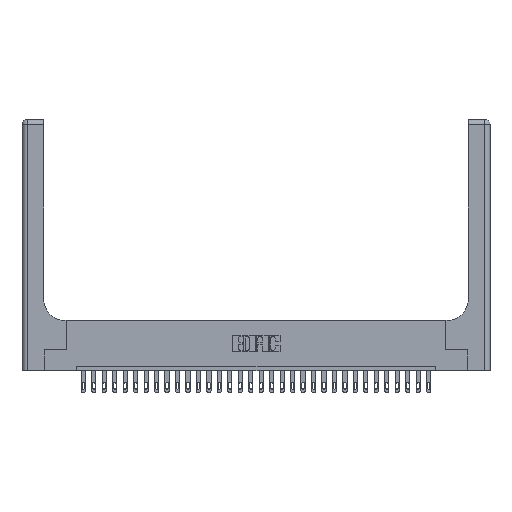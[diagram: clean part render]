
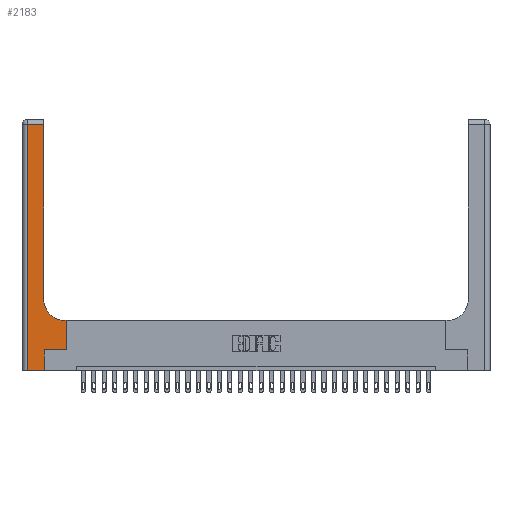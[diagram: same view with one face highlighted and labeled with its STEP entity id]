
A CAD part, top view. The second image highlights one B-rep face of the part: STEP entity #2183.
In plain terms, the highlighted planar face has unit normal (0, 0, 1).
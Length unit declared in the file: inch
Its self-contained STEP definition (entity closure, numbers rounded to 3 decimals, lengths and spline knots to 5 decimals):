
#355 = VERTEX_POINT ( 'NONE', #3595 ) ;
#551 = LINE ( 'NONE', #9182, #11327 ) ;
#972 = ORIENTED_EDGE ( 'NONE', *, *, #5209, .T. ) ;
#1092 = LINE ( 'NONE', #9715, #8685 ) ;
#1615 = VECTOR ( 'NONE', #13445, 39.37008 ) ;
#1952 = CARTESIAN_POINT ( 'NONE',  ( 0.528, 0.25, 0.37 ) ) ;
#2121 = VERTEX_POINT ( 'NONE', #25335 ) ;
#2130 = DIRECTION ( 'NONE',  ( 1., 0., 0. ) ) ;
#2183 = ADVANCED_FACE ( 'NONE', ( #14307 ), #10513, .F. ) ;
#2199 = LINE ( 'NONE', #19317, #1615 ) ;
#2420 = CIRCLE ( 'NONE', #7799, 0.25 ) ;
#2628 = CARTESIAN_POINT ( 'NONE',  ( 0.528, 0.6, 0.37 ) ) ;
#2995 = ORIENTED_EDGE ( 'NONE', *, *, #22222, .T. ) ;
#2997 = LINE ( 'NONE', #15668, #6789 ) ;
#3107 = ORIENTED_EDGE ( 'NONE', *, *, #4448, .T. ) ;
#3123 = VERTEX_POINT ( 'NONE', #27421 ) ;
#3236 = VERTEX_POINT ( 'NONE', #13981 ) ;
#3387 = VERTEX_POINT ( 'NONE', #27386 ) ;
#3470 = CARTESIAN_POINT ( 'NONE',  ( 0.06, 0., 0.37 ) ) ;
#3595 = CARTESIAN_POINT ( 'NONE',  ( 0.51, 0.6, 0.37 ) ) ;
#3900 = CARTESIAN_POINT ( 'NONE',  ( 0.26, 3., 0.37 ) ) ;
#4389 = LINE ( 'NONE', #23306, #5181 ) ;
#4448 = EDGE_CURVE ( 'NONE', #3236, #3387, #16285, .T. ) ;
#4560 = EDGE_CURVE ( 'NONE', #355, #3236, #2420, .T. ) ;
#5181 = VECTOR ( 'NONE', #2130, 39.37008 ) ;
#5209 = EDGE_CURVE ( 'NONE', #23020, #355, #1092, .T. ) ;
#5380 = CARTESIAN_POINT ( 'NONE',  ( 0., 0., 0.37 ) ) ;
#5548 = ORIENTED_EDGE ( 'NONE', *, *, #22301, .T. ) ;
#5926 = VECTOR ( 'NONE', #22434, 39.37008 ) ;
#6789 = VECTOR ( 'NONE', #6935, 39.37008 ) ;
#6935 = DIRECTION ( 'NONE',  ( 0., 1., 0. ) ) ;
#7799 = AXIS2_PLACEMENT_3D ( 'NONE', #12029, #18443, #25027 ) ;
#7832 = CARTESIAN_POINT ( 'NONE',  ( 0., 3., 0.37 ) ) ;
#8685 = VECTOR ( 'NONE', #26753, 39.37008 ) ;
#8744 = LINE ( 'NONE', #1952, #20261 ) ;
#9182 = CARTESIAN_POINT ( 'NONE',  ( 0.06, 3., 0.37 ) ) ;
#9715 = CARTESIAN_POINT ( 'NONE',  ( 0.26, 0.6, 0.37 ) ) ;
#10513 = PLANE ( 'NONE',  #22110 ) ;
#10843 = EDGE_LOOP ( 'NONE', ( #3107, #25545, #2995, #20939, #13868, #22587, #5548, #972, #20157 ) ) ;
#11242 = VERTEX_POINT ( 'NONE', #13405 ) ;
#11327 = VECTOR ( 'NONE', #15640, 39.37008 ) ;
#12029 = CARTESIAN_POINT ( 'NONE',  ( 0.51, 0.85, 0.37 ) ) ;
#12085 = VERTEX_POINT ( 'NONE', #26296 ) ;
#13405 = CARTESIAN_POINT ( 'NONE',  ( 0.528, 0.25, 0.37 ) ) ;
#13445 = DIRECTION ( 'NONE',  ( -1., 0., 0. ) ) ;
#13868 = ORIENTED_EDGE ( 'NONE', *, *, #20832, .T. ) ;
#13940 = LINE ( 'NONE', #5380, #5926 ) ;
#13981 = CARTESIAN_POINT ( 'NONE',  ( 0.26, 0.85, 0.37 ) ) ;
#14307 = FACE_OUTER_BOUND ( 'NONE', #10843, .T. ) ;
#14765 = VERTEX_POINT ( 'NONE', #3470 ) ;
#15640 = DIRECTION ( 'NONE',  ( 0., -1., 0. ) ) ;
#15668 = CARTESIAN_POINT ( 'NONE',  ( 0.265, 0., 0.37 ) ) ;
#16285 = LINE ( 'NONE', #3900, #24372 ) ;
#16416 = DIRECTION ( 'NONE',  ( 0., 0., -1. ) ) ;
#18061 = EDGE_CURVE ( 'NONE', #3387, #3123, #2199, .T. ) ;
#18349 = DIRECTION ( 'NONE',  ( 0., 1., 0. ) ) ;
#18443 = DIRECTION ( 'NONE',  ( 0., 0., -1. ) ) ;
#19317 = CARTESIAN_POINT ( 'NONE',  ( 0., 2.94, 0.37 ) ) ;
#19501 = DIRECTION ( 'NONE',  ( 0., 1., 0. ) ) ;
#20157 = ORIENTED_EDGE ( 'NONE', *, *, #4560, .T. ) ;
#20261 = VECTOR ( 'NONE', #19501, 39.37008 ) ;
#20832 = EDGE_CURVE ( 'NONE', #2121, #12085, #2997, .T. ) ;
#20939 = ORIENTED_EDGE ( 'NONE', *, *, #26766, .T. ) ;
#22110 = AXIS2_PLACEMENT_3D ( 'NONE', #7832, #16416, #24930 ) ;
#22222 = EDGE_CURVE ( 'NONE', #3123, #14765, #551, .T. ) ;
#22301 = EDGE_CURVE ( 'NONE', #11242, #23020, #8744, .T. ) ;
#22434 = DIRECTION ( 'NONE',  ( 1., 0., 0. ) ) ;
#22587 = ORIENTED_EDGE ( 'NONE', *, *, #24794, .T. ) ;
#23020 = VERTEX_POINT ( 'NONE', #2628 ) ;
#23306 = CARTESIAN_POINT ( 'NONE',  ( 0.265, 0.25, 0.37 ) ) ;
#24372 = VECTOR ( 'NONE', #18349, 39.37008 ) ;
#24794 = EDGE_CURVE ( 'NONE', #12085, #11242, #4389, .T. ) ;
#24930 = DIRECTION ( 'NONE',  ( -1., 0., 0. ) ) ;
#25027 = DIRECTION ( 'NONE',  ( 1., 0., 0. ) ) ;
#25335 = CARTESIAN_POINT ( 'NONE',  ( 0.265, 0., 0.37 ) ) ;
#25545 = ORIENTED_EDGE ( 'NONE', *, *, #18061, .T. ) ;
#26296 = CARTESIAN_POINT ( 'NONE',  ( 0.265, 0.25, 0.37 ) ) ;
#26753 = DIRECTION ( 'NONE',  ( -1., 0., 0. ) ) ;
#26766 = EDGE_CURVE ( 'NONE', #14765, #2121, #13940, .T. ) ;
#27386 = CARTESIAN_POINT ( 'NONE',  ( 0.26, 2.94, 0.37 ) ) ;
#27421 = CARTESIAN_POINT ( 'NONE',  ( 0.06, 2.94, 0.37 ) ) ;
